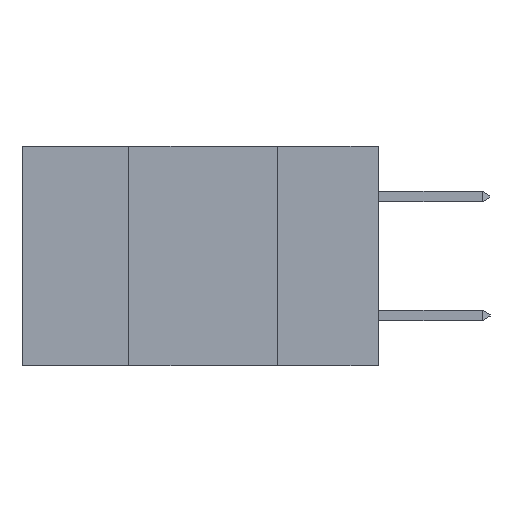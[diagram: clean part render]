
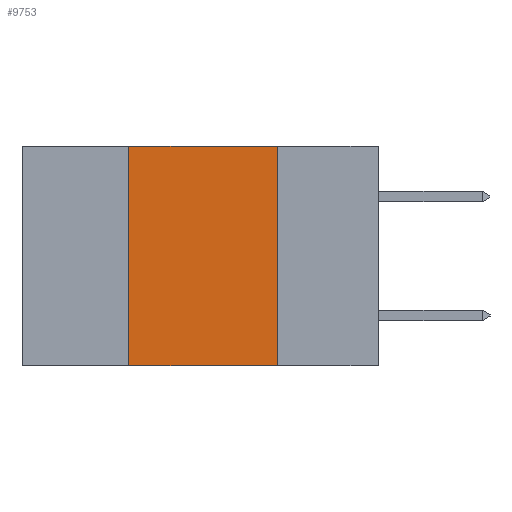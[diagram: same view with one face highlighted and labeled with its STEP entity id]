
A CAD part, left-side view. The second image highlights one B-rep face of the part: STEP entity #9753.
In plain terms, the highlighted planar face has unit normal (-1, 0, 0).
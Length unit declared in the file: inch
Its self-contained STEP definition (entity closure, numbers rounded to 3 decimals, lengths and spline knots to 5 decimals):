
#127 = DIRECTION ( 'NONE',  ( 0., 0., 1. ) ) ;
#202 = LINE ( 'NONE', #12347, #8142 ) ;
#343 = DIRECTION ( 'NONE',  ( 0., 0., -1. ) ) ;
#520 = DIRECTION ( 'NONE',  ( 1., 0., 0. ) ) ;
#588 = PLANE ( 'NONE',  #3736 ) ;
#678 = VERTEX_POINT ( 'NONE', #12316 ) ;
#796 = CARTESIAN_POINT ( 'NONE',  ( 0., 0.6, 0. ) ) ;
#1057 = LINE ( 'NONE', #4847, #12222 ) ;
#1604 = EDGE_CURVE ( 'NONE', #13067, #678, #202, .T. ) ;
#3077 = ORIENTED_EDGE ( 'NONE', *, *, #4003, .T. ) ;
#3736 = AXIS2_PLACEMENT_3D ( 'NONE', #796, #520, #343 ) ;
#3878 = ORIENTED_EDGE ( 'NONE', *, *, #1604, .F. ) ;
#4003 = EDGE_CURVE ( 'NONE', #13067, #12006, #6358, .T. ) ;
#4757 = DIRECTION ( 'NONE',  ( 0., 0., -1. ) ) ;
#4847 = CARTESIAN_POINT ( 'NONE',  ( 0., 0.17, -0.37 ) ) ;
#5182 = LINE ( 'NONE', #9056, #10294 ) ;
#6358 = LINE ( 'NONE', #11694, #11755 ) ;
#6784 = CARTESIAN_POINT ( 'NONE',  ( 0., 0.17, 0. ) ) ;
#7479 = CARTESIAN_POINT ( 'NONE',  ( 0., 0.42, -0.37 ) ) ;
#8142 = VECTOR ( 'NONE', #127, 39.37008 ) ;
#8384 = EDGE_CURVE ( 'NONE', #11387, #12006, #1057, .T. ) ;
#8458 = CARTESIAN_POINT ( 'NONE',  ( 0., 0.17, -0.37 ) ) ;
#8953 = DIRECTION ( 'NONE',  ( 0., -1., 0. ) ) ;
#9056 = CARTESIAN_POINT ( 'NONE',  ( 0., 0.6, 0. ) ) ;
#9753 = ADVANCED_FACE ( 'NONE', ( #12512 ), #588, .F. ) ;
#10294 = VECTOR ( 'NONE', #8953, 39.37008 ) ;
#11387 = VERTEX_POINT ( 'NONE', #6784 ) ;
#11694 = CARTESIAN_POINT ( 'NONE',  ( 0., 0.6, -0.37 ) ) ;
#11755 = VECTOR ( 'NONE', #11940, 39.37008 ) ;
#11844 = EDGE_LOOP ( 'NONE', ( #12607, #12966, #3878, #3077 ) ) ;
#11940 = DIRECTION ( 'NONE',  ( 0., -1., 0. ) ) ;
#12006 = VERTEX_POINT ( 'NONE', #8458 ) ;
#12222 = VECTOR ( 'NONE', #4757, 39.37008 ) ;
#12316 = CARTESIAN_POINT ( 'NONE',  ( 0., 0.42, 0. ) ) ;
#12347 = CARTESIAN_POINT ( 'NONE',  ( 0., 0.42, -0.37 ) ) ;
#12512 = FACE_OUTER_BOUND ( 'NONE', #11844, .T. ) ;
#12607 = ORIENTED_EDGE ( 'NONE', *, *, #8384, .F. ) ;
#12966 = ORIENTED_EDGE ( 'NONE', *, *, #12971, .F. ) ;
#12971 = EDGE_CURVE ( 'NONE', #678, #11387, #5182, .T. ) ;
#13067 = VERTEX_POINT ( 'NONE', #7479 ) ;
